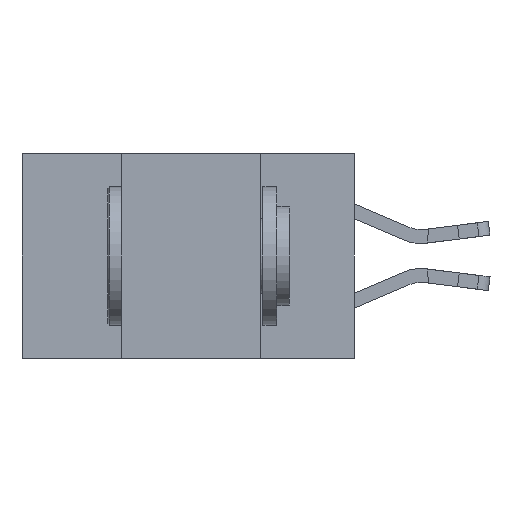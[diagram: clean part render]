
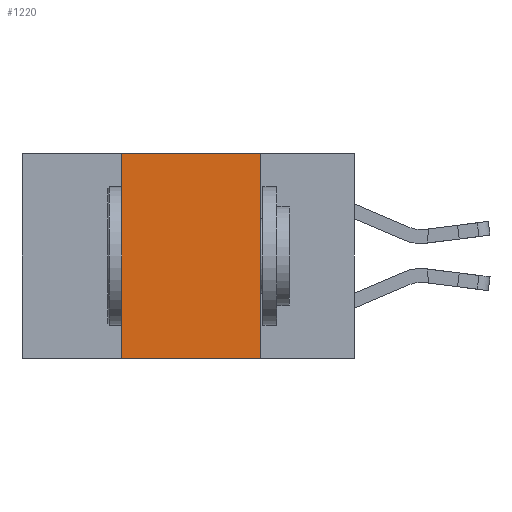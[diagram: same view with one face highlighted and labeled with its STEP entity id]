
A CAD part, left-side view. The second image highlights one B-rep face of the part: STEP entity #1220.
In plain terms, the highlighted planar face has unit normal (-1, 0, 0).
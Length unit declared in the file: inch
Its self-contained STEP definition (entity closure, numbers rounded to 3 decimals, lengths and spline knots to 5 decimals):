
#637 = VECTOR ( 'NONE', #10783, 39.37008 ) ;
#1100 = CARTESIAN_POINT ( 'NONE',  ( 0., 0.42, 0. ) ) ;
#1177 = VECTOR ( 'NONE', #13463, 39.37008 ) ;
#1220 = ADVANCED_FACE ( 'NONE', ( #11609 ), #12262, .F. ) ;
#1239 = VERTEX_POINT ( 'NONE', #4298 ) ;
#2315 = EDGE_CURVE ( 'NONE', #1239, #8276, #11398, .T. ) ;
#2570 = VERTEX_POINT ( 'NONE', #13347 ) ;
#3892 = CARTESIAN_POINT ( 'NONE',  ( 0., 0.17, -0.37 ) ) ;
#3982 = EDGE_CURVE ( 'NONE', #1239, #6698, #13131, .T. ) ;
#4298 = CARTESIAN_POINT ( 'NONE',  ( 0., 0.42, -0.37 ) ) ;
#4764 = EDGE_CURVE ( 'NONE', #6698, #2570, #9589, .T. ) ;
#5294 = DIRECTION ( 'NONE',  ( 0., 0., -1. ) ) ;
#5607 = ORIENTED_EDGE ( 'NONE', *, *, #2315, .T. ) ;
#5985 = ORIENTED_EDGE ( 'NONE', *, *, #7167, .F. ) ;
#6487 = DIRECTION ( 'NONE',  ( 0., -1., 0. ) ) ;
#6698 = VERTEX_POINT ( 'NONE', #1100 ) ;
#7167 = EDGE_CURVE ( 'NONE', #2570, #8276, #12155, .T. ) ;
#8276 = VERTEX_POINT ( 'NONE', #9359 ) ;
#8784 = ORIENTED_EDGE ( 'NONE', *, *, #3982, .F. ) ;
#9007 = DIRECTION ( 'NONE',  ( 0., 0., -1. ) ) ;
#9040 = DIRECTION ( 'NONE',  ( 1., 0., 0. ) ) ;
#9359 = CARTESIAN_POINT ( 'NONE',  ( 0., 0.17, -0.37 ) ) ;
#9589 = LINE ( 'NONE', #10815, #637 ) ;
#10030 = CARTESIAN_POINT ( 'NONE',  ( 0., 0.6, -0.37 ) ) ;
#10783 = DIRECTION ( 'NONE',  ( 0., -1., 0. ) ) ;
#10815 = CARTESIAN_POINT ( 'NONE',  ( 0., 0.6, 0. ) ) ;
#11176 = EDGE_LOOP ( 'NONE', ( #5985, #11752, #8784, #5607 ) ) ;
#11398 = LINE ( 'NONE', #10030, #12132 ) ;
#11609 = FACE_OUTER_BOUND ( 'NONE', #11176, .T. ) ;
#11752 = ORIENTED_EDGE ( 'NONE', *, *, #4764, .F. ) ;
#11769 = VECTOR ( 'NONE', #5294, 39.37008 ) ;
#12132 = VECTOR ( 'NONE', #6487, 39.37008 ) ;
#12155 = LINE ( 'NONE', #3892, #11769 ) ;
#12200 = CARTESIAN_POINT ( 'NONE',  ( 0., 0.6, 0. ) ) ;
#12262 = PLANE ( 'NONE',  #14024 ) ;
#13131 = LINE ( 'NONE', #13553, #1177 ) ;
#13347 = CARTESIAN_POINT ( 'NONE',  ( 0., 0.17, 0. ) ) ;
#13463 = DIRECTION ( 'NONE',  ( 0., 0., 1. ) ) ;
#13553 = CARTESIAN_POINT ( 'NONE',  ( 0., 0.42, -0.37 ) ) ;
#14024 = AXIS2_PLACEMENT_3D ( 'NONE', #12200, #9040, #9007 ) ;
